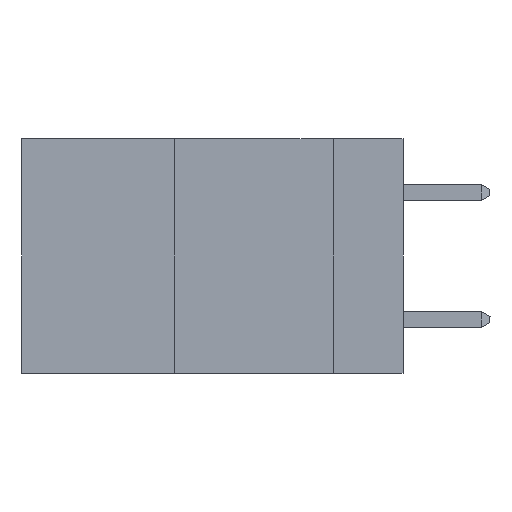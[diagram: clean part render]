
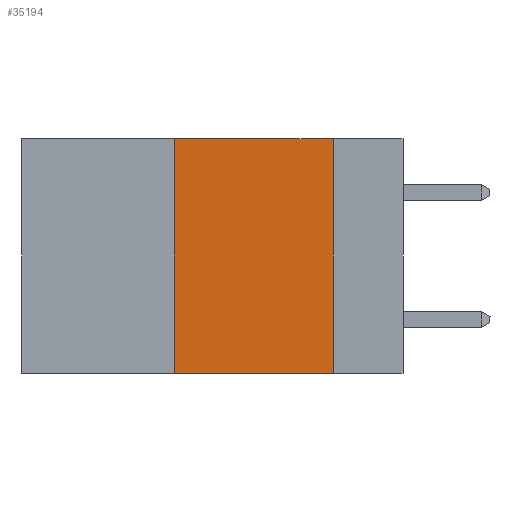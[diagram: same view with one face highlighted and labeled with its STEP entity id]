
A CAD part, left-side view. The second image highlights one B-rep face of the part: STEP entity #35194.
In plain terms, the highlighted planar face has unit normal (-1, 0, 0).
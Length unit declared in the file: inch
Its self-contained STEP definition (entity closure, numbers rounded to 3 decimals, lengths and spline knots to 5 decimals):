
#234 = VERTEX_POINT ( 'NONE', #34746 ) ;
#2687 = CARTESIAN_POINT ( 'NONE',  ( 0., 0.36, 0. ) ) ;
#3022 = EDGE_CURVE ( 'NONE', #21519, #39882, #5484, .T. ) ;
#3082 = ORIENTED_EDGE ( 'NONE', *, *, #9362, .F. ) ;
#3403 = LINE ( 'NONE', #26826, #24687 ) ;
#4707 = LINE ( 'NONE', #19677, #25499 ) ;
#5085 = ORIENTED_EDGE ( 'NONE', *, *, #14168, .F. ) ;
#5484 = LINE ( 'NONE', #37715, #33001 ) ;
#9362 = EDGE_CURVE ( 'NONE', #18015, #21519, #38334, .T. ) ;
#9567 = EDGE_LOOP ( 'NONE', ( #5085, #23926, #3082, #34214 ) ) ;
#14168 = EDGE_CURVE ( 'NONE', #39882, #234, #4707, .T. ) ;
#14874 = CARTESIAN_POINT ( 'NONE',  ( 0., 0.6, 0. ) ) ;
#17959 = DIRECTION ( 'NONE',  ( 0., -1., 0. ) ) ;
#17969 = FACE_OUTER_BOUND ( 'NONE', #9567, .T. ) ;
#18015 = VERTEX_POINT ( 'NONE', #24260 ) ;
#18376 = DIRECTION ( 'NONE',  ( 0., 0., -1. ) ) ;
#19677 = CARTESIAN_POINT ( 'NONE',  ( 0., 0.11, 0. ) ) ;
#21207 = VECTOR ( 'NONE', #29391, 39.37008 ) ;
#21519 = VERTEX_POINT ( 'NONE', #27033 ) ;
#23926 = ORIENTED_EDGE ( 'NONE', *, *, #3022, .F. ) ;
#24260 = CARTESIAN_POINT ( 'NONE',  ( 0., 0.36, -0.37 ) ) ;
#24687 = VECTOR ( 'NONE', #30298, 39.37008 ) ;
#25499 = VECTOR ( 'NONE', #36103, 39.37008 ) ;
#26826 = CARTESIAN_POINT ( 'NONE',  ( 0., 0.6, -0.37 ) ) ;
#27033 = CARTESIAN_POINT ( 'NONE',  ( 0., 0.36, 0. ) ) ;
#29391 = DIRECTION ( 'NONE',  ( 0., 0., 1. ) ) ;
#30298 = DIRECTION ( 'NONE',  ( 0., -1., 0. ) ) ;
#30540 = EDGE_CURVE ( 'NONE', #18015, #234, #3403, .T. ) ;
#31387 = AXIS2_PLACEMENT_3D ( 'NONE', #14874, #31597, #18376 ) ;
#31597 = DIRECTION ( 'NONE',  ( 1., 0., 0. ) ) ;
#32052 = PLANE ( 'NONE',  #31387 ) ;
#33001 = VECTOR ( 'NONE', #17959, 39.37008 ) ;
#34214 = ORIENTED_EDGE ( 'NONE', *, *, #30540, .T. ) ;
#34746 = CARTESIAN_POINT ( 'NONE',  ( 0., 0.11, -0.37 ) ) ;
#35194 = ADVANCED_FACE ( 'NONE', ( #17969 ), #32052, .F. ) ;
#36103 = DIRECTION ( 'NONE',  ( 0., 0., -1. ) ) ;
#37715 = CARTESIAN_POINT ( 'NONE',  ( 0., 0.6, 0. ) ) ;
#38334 = LINE ( 'NONE', #2687, #21207 ) ;
#39882 = VERTEX_POINT ( 'NONE', #40633 ) ;
#40633 = CARTESIAN_POINT ( 'NONE',  ( 0., 0.11, 0. ) ) ;
